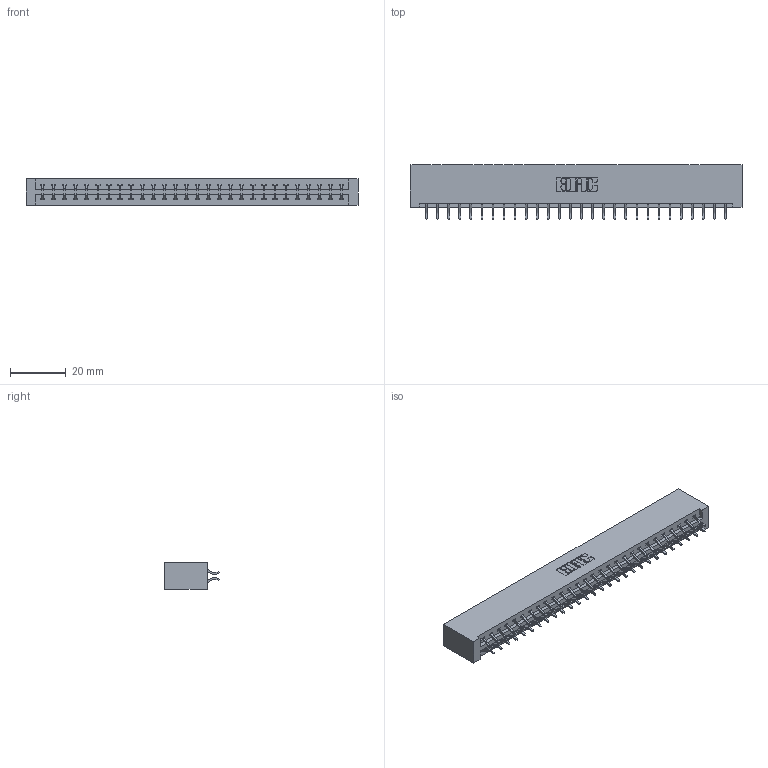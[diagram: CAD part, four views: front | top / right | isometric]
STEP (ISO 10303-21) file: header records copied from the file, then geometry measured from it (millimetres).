
FILE_DESCRIPTION (( 'STEP AP203' ), '1' );
FILE_NAME ('337-056-556-201.STEP', '2018-08-10T03:38:52', ( '' ), ( '' ), 'SwSTEP 2.0', 'SolidWorks 2016', '' );
FILE_SCHEMA (( 'CONFIG_CONTROL_DESIGN' ));
Length unit declared in the file: inch
Products named in the file (3): 337 Part_No Mounting Lugs; 345-292-001_556 Tail; 337-056-556-201
Assembly tree (57 placements, depth 2):
  337-056-556-201
    337 Part_No Mounting Lugs
    345-292-001_556 Tail  x56
Bounding box: 118.82 x 19.57 x 9.4 mm (x, y, z)
Volume: 13094.5 mm3; surface area: 14664.4 mm2
Topology: 57 solids, 57 shells, 3466 faces, 10311 edges, 6798 vertices
Faces by surface type: plane 2418, cylinder 1048
Entity records: 23463 total; most frequent: CARTESIAN_POINT 3978, ORIENTED_EDGE 3902, DIRECTION 3391, EDGE_CURVE 1951, VECTOR 1823, LINE 1823, VERTEX_POINT 1298, AXIS2_PLACEMENT_3D 784
